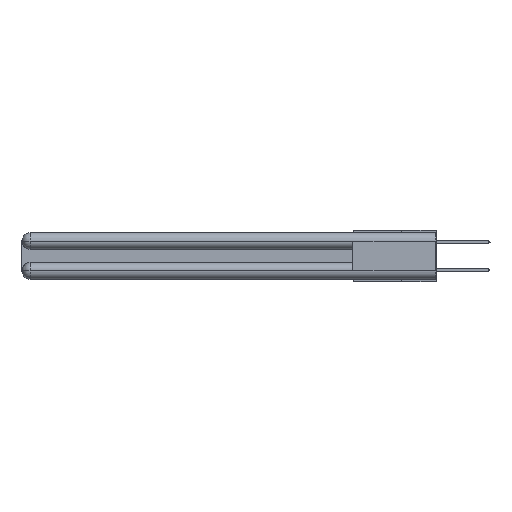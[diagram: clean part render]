
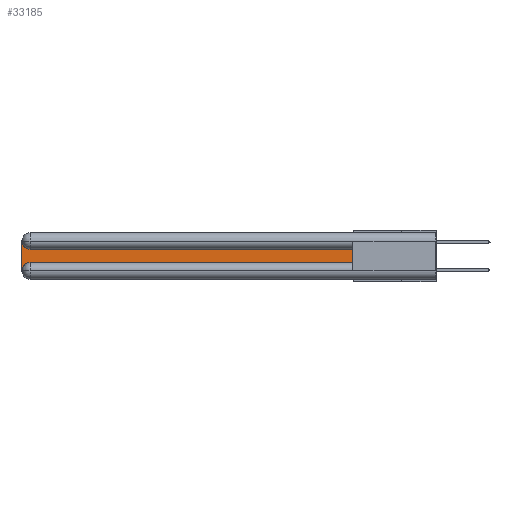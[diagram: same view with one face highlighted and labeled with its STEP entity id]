
A CAD part, left-side view. The second image highlights one B-rep face of the part: STEP entity #33185.
In plain terms, the highlighted planar face has unit normal (-1, 0, 0).
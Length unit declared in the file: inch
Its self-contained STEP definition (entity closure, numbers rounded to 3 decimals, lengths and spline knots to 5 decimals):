
#473 = DIRECTION ( 'NONE',  ( 1., 0., 0. ) ) ;
#680 = ORIENTED_EDGE ( 'NONE', *, *, #26362, .T. ) ;
#782 = CARTESIAN_POINT ( 'NONE',  ( 0.075, 0.6, -0.2175 ) ) ;
#885 = VECTOR ( 'NONE', #16187, 39.37008 ) ;
#1968 = EDGE_CURVE ( 'NONE', #16996, #21926, #14393, .T. ) ;
#2941 = LINE ( 'NONE', #21824, #885 ) ;
#4022 = CARTESIAN_POINT ( 'NONE',  ( 0.075, 0.6, -0.2175 ) ) ;
#6862 = ORIENTED_EDGE ( 'NONE', *, *, #14437, .T. ) ;
#7089 = ORIENTED_EDGE ( 'NONE', *, *, #33908, .T. ) ;
#7242 = LINE ( 'NONE', #7248, #23154 ) ;
#7248 = CARTESIAN_POINT ( 'NONE',  ( 0.075, 0.6, -0.2175 ) ) ;
#9222 = CARTESIAN_POINT ( 'NONE',  ( 0.075, 2.94, -0.2775 ) ) ;
#9914 = EDGE_LOOP ( 'NONE', ( #680, #24371, #6862, #7089, #10333, #14643 ) ) ;
#10333 = ORIENTED_EDGE ( 'NONE', *, *, #25639, .T. ) ;
#11458 = VECTOR ( 'NONE', #20141, 39.37008 ) ;
#14287 = DIRECTION ( 'NONE',  ( 0., 1., 0. ) ) ;
#14393 = LINE ( 'NONE', #4022, #11458 ) ;
#14437 = EDGE_CURVE ( 'NONE', #18721, #17372, #2941, .T. ) ;
#14643 = ORIENTED_EDGE ( 'NONE', *, *, #1968, .T. ) ;
#14709 = CIRCLE ( 'NONE', #34271, 0.06 ) ;
#14748 = VECTOR ( 'NONE', #14287, 39.37008 ) ;
#14809 = EDGE_CURVE ( 'NONE', #18874, #18721, #28437, .T. ) ;
#15235 = DIRECTION ( 'NONE',  ( 0., 0., -1. ) ) ;
#16187 = DIRECTION ( 'NONE',  ( 0., 0., -1. ) ) ;
#16271 = CARTESIAN_POINT ( 'NONE',  ( 0.075, 2.94, -0.1225 ) ) ;
#16996 = VERTEX_POINT ( 'NONE', #782 ) ;
#17372 = VERTEX_POINT ( 'NONE', #30158 ) ;
#17799 = DIRECTION ( 'NONE',  ( 1., 0., 0. ) ) ;
#18378 = DIRECTION ( 'NONE',  ( 0., 0., -1. ) ) ;
#18721 = VERTEX_POINT ( 'NONE', #26474 ) ;
#18874 = VERTEX_POINT ( 'NONE', #16271 ) ;
#19821 = FACE_OUTER_BOUND ( 'NONE', #9914, .T. ) ;
#20141 = DIRECTION ( 'NONE',  ( 0., 0., 1. ) ) ;
#20593 = DIRECTION ( 'NONE',  ( 0., -1., 0. ) ) ;
#20628 = AXIS2_PLACEMENT_3D ( 'NONE', #21434, #21323, #18378 ) ;
#21008 = CARTESIAN_POINT ( 'NONE',  ( 0.075, 0.6, -0.1225 ) ) ;
#21323 = DIRECTION ( 'NONE',  ( 1., 0., 0. ) ) ;
#21434 = CARTESIAN_POINT ( 'NONE',  ( 0.075, 3., -0.1225 ) ) ;
#21824 = CARTESIAN_POINT ( 'NONE',  ( 0.075, 3., -0.2175 ) ) ;
#21849 = DIRECTION ( 'NONE',  ( 0., 0., -1. ) ) ;
#21926 = VERTEX_POINT ( 'NONE', #21008 ) ;
#22283 = LINE ( 'NONE', #30187, #14748 ) ;
#23154 = VECTOR ( 'NONE', #20593, 39.37008 ) ;
#23421 = CARTESIAN_POINT ( 'NONE',  ( 0.075, 2.94, -0.0625 ) ) ;
#24371 = ORIENTED_EDGE ( 'NONE', *, *, #14809, .T. ) ;
#25639 = EDGE_CURVE ( 'NONE', #30966, #16996, #7242, .T. ) ;
#26362 = EDGE_CURVE ( 'NONE', #21926, #18874, #22283, .T. ) ;
#26474 = CARTESIAN_POINT ( 'NONE',  ( 0.075, 3., -0.0625 ) ) ;
#26698 = PLANE ( 'NONE',  #20628 ) ;
#28437 = CIRCLE ( 'NONE', #33926, 0.06 ) ;
#30158 = CARTESIAN_POINT ( 'NONE',  ( 0.075, 3., -0.2775 ) ) ;
#30187 = CARTESIAN_POINT ( 'NONE',  ( 0.075, 0.6, -0.1225 ) ) ;
#30966 = VERTEX_POINT ( 'NONE', #33675 ) ;
#33185 = ADVANCED_FACE ( 'NONE', ( #19821 ), #26698, .F. ) ;
#33675 = CARTESIAN_POINT ( 'NONE',  ( 0.075, 2.94, -0.2175 ) ) ;
#33908 = EDGE_CURVE ( 'NONE', #17372, #30966, #14709, .T. ) ;
#33926 = AXIS2_PLACEMENT_3D ( 'NONE', #23421, #17799, #15235 ) ;
#34271 = AXIS2_PLACEMENT_3D ( 'NONE', #9222, #473, #21849 ) ;
